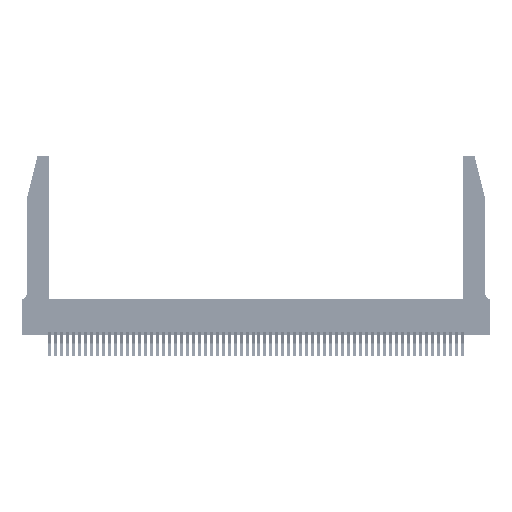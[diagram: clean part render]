
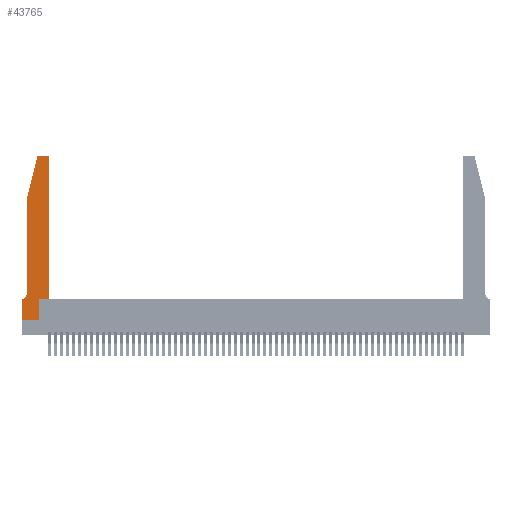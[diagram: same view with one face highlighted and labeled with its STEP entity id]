
A CAD part, top view. The second image highlights one B-rep face of the part: STEP entity #43765.
In plain terms, the highlighted planar face has unit normal (0, 0, 1).
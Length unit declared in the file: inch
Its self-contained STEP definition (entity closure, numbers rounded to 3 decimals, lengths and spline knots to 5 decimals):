
#1650 = CIRCLE ( 'NONE', #48432, 0.07 ) ;
#1701 = CARTESIAN_POINT ( 'NONE',  ( 0.25487, 2.72718, 0.37 ) ) ;
#2907 = VECTOR ( 'NONE', #38109, 39.37008 ) ;
#3611 = LINE ( 'NONE', #40424, #30001 ) ;
#4774 = ORIENTED_EDGE ( 'NONE', *, *, #10449, .T. ) ;
#5428 = VERTEX_POINT ( 'NONE', #1701 ) ;
#5796 = ORIENTED_EDGE ( 'NONE', *, *, #35148, .T. ) ;
#6110 = VECTOR ( 'NONE', #34499, 39.37008 ) ;
#6294 = ORIENTED_EDGE ( 'NONE', *, *, #17720, .T. ) ;
#7890 = VERTEX_POINT ( 'NONE', #23290 ) ;
#7939 = ORIENTED_EDGE ( 'NONE', *, *, #19952, .T. ) ;
#8079 = CARTESIAN_POINT ( 'NONE',  ( 0., 0.35, 0.37 ) ) ;
#8373 = CARTESIAN_POINT ( 'NONE',  ( 0., 0.35, 0.37 ) ) ;
#9248 = VECTOR ( 'NONE', #18853, 39.37008 ) ;
#9257 = AXIS2_PLACEMENT_3D ( 'NONE', #19290, #45790, #23870 ) ;
#10449 = EDGE_CURVE ( 'NONE', #30890, #24434, #25084, .T. ) ;
#11018 = CARTESIAN_POINT ( 'NONE',  ( 0.4505, 0.35, 0.37 ) ) ;
#11156 = VERTEX_POINT ( 'NONE', #47682 ) ;
#12331 = AXIS2_PLACEMENT_3D ( 'NONE', #15056, #23778, #18841 ) ;
#12369 = PLANE ( 'NONE',  #45877 ) ;
#12887 = CARTESIAN_POINT ( 'NONE',  ( 0.4205, 2.75, 0.37 ) ) ;
#13265 = VERTEX_POINT ( 'NONE', #41209 ) ;
#14393 = EDGE_CURVE ( 'NONE', #37479, #23660, #1650, .T. ) ;
#14399 = LINE ( 'NONE', #33569, #2907 ) ;
#14566 = VECTOR ( 'NONE', #15177, 39.37008 ) ;
#14659 = DIRECTION ( 'NONE',  ( 0., -1., 0. ) ) ;
#14742 = ORIENTED_EDGE ( 'NONE', *, *, #29543, .T. ) ;
#15056 = CARTESIAN_POINT ( 'NONE',  ( 0.284, 2.72, 0.37 ) ) ;
#15161 = ORIENTED_EDGE ( 'NONE', *, *, #37620, .T. ) ;
#15177 = DIRECTION ( 'NONE',  ( 0., 1., 0. ) ) ;
#15316 = LINE ( 'NONE', #29468, #33639 ) ;
#15546 = CARTESIAN_POINT ( 'NONE',  ( 0.0755, 2., 0.37 ) ) ;
#15701 = ORIENTED_EDGE ( 'NONE', *, *, #47760, .T. ) ;
#17720 = EDGE_CURVE ( 'NONE', #7890, #37479, #26825, .T. ) ;
#17823 = CARTESIAN_POINT ( 'NONE',  ( 0., 0., 0.37 ) ) ;
#17863 = EDGE_CURVE ( 'NONE', #11156, #40596, #15316, .T. ) ;
#17932 = LINE ( 'NONE', #49998, #14566 ) ;
#18460 = ORIENTED_EDGE ( 'NONE', *, *, #36901, .T. ) ;
#18503 = ORIENTED_EDGE ( 'NONE', *, *, #42354, .T. ) ;
#18841 = DIRECTION ( 'NONE',  ( 1., 0., 0. ) ) ;
#18853 = DIRECTION ( 'NONE',  ( 0., -1., 0. ) ) ;
#19290 = CARTESIAN_POINT ( 'NONE',  ( 0.4205, 2.72, 0.37 ) ) ;
#19952 = EDGE_CURVE ( 'NONE', #23660, #39487, #14399, .T. ) ;
#20032 = EDGE_LOOP ( 'NONE', ( #5796, #18460, #15161, #6294, #37038, #7939, #15701, #4774, #34388, #26425, #14742, #18503 ) ) ;
#20660 = DIRECTION ( 'NONE',  ( 0., 0., 1. ) ) ;
#20765 = CARTESIAN_POINT ( 'NONE',  ( 0.2865, 0.35, 0.37 ) ) ;
#23290 = CARTESIAN_POINT ( 'NONE',  ( 0.0755, 2., 0.37 ) ) ;
#23589 = CARTESIAN_POINT ( 'NONE',  ( 0.0055, 0.35, 0.37 ) ) ;
#23660 = VERTEX_POINT ( 'NONE', #23589 ) ;
#23778 = DIRECTION ( 'NONE',  ( 0., 0., 1. ) ) ;
#23870 = DIRECTION ( 'NONE',  ( 1., 0., 0. ) ) ;
#24434 = VERTEX_POINT ( 'NONE', #51154 ) ;
#25084 = LINE ( 'NONE', #17823, #6110 ) ;
#26360 = VERTEX_POINT ( 'NONE', #12887 ) ;
#26425 = ORIENTED_EDGE ( 'NONE', *, *, #17863, .T. ) ;
#26825 = LINE ( 'NONE', #49326, #9248 ) ;
#28053 = DIRECTION ( 'NONE',  ( -1., 0., 0. ) ) ;
#29468 = CARTESIAN_POINT ( 'NONE',  ( 0.4505, 0.35, 0.37 ) ) ;
#29543 = EDGE_CURVE ( 'NONE', #40596, #13265, #17932, .T. ) ;
#30001 = VECTOR ( 'NONE', #14659, 39.37008 ) ;
#30333 = EDGE_CURVE ( 'NONE', #24434, #11156, #36844, .T. ) ;
#30449 = VECTOR ( 'NONE', #32215, 39.37008 ) ;
#30890 = VERTEX_POINT ( 'NONE', #54794 ) ;
#31772 = VERTEX_POINT ( 'NONE', #43713 ) ;
#32215 = DIRECTION ( 'NONE',  ( -0.239, -0.971, 0. ) ) ;
#33274 = DIRECTION ( 'NONE',  ( 0., 1., 0. ) ) ;
#33569 = CARTESIAN_POINT ( 'NONE',  ( 0.0755, 0.35, 0.37 ) ) ;
#33639 = VECTOR ( 'NONE', #53867, 39.37008 ) ;
#34146 = VECTOR ( 'NONE', #33274, 39.37008 ) ;
#34388 = ORIENTED_EDGE ( 'NONE', *, *, #30333, .T. ) ;
#34499 = DIRECTION ( 'NONE',  ( 1., 0., 0. ) ) ;
#35148 = EDGE_CURVE ( 'NONE', #26360, #31772, #46287, .T. ) ;
#36403 = CARTESIAN_POINT ( 'NONE',  ( 0.0055, 0.42, 0.37 ) ) ;
#36844 = LINE ( 'NONE', #20765, #34146 ) ;
#36901 = EDGE_CURVE ( 'NONE', #31772, #5428, #52225, .T. ) ;
#37038 = ORIENTED_EDGE ( 'NONE', *, *, #14393, .T. ) ;
#37479 = VERTEX_POINT ( 'NONE', #40373 ) ;
#37620 = EDGE_CURVE ( 'NONE', #5428, #7890, #41949, .T. ) ;
#38109 = DIRECTION ( 'NONE',  ( -1., 0., 0. ) ) ;
#39487 = VERTEX_POINT ( 'NONE', #8079 ) ;
#40373 = CARTESIAN_POINT ( 'NONE',  ( 0.0755, 0.42, 0.37 ) ) ;
#40424 = CARTESIAN_POINT ( 'NONE',  ( 0., 0., 0.37 ) ) ;
#40596 = VERTEX_POINT ( 'NONE', #11018 ) ;
#41209 = CARTESIAN_POINT ( 'NONE',  ( 0.4505, 2.72, 0.37 ) ) ;
#41492 = CIRCLE ( 'NONE', #9257, 0.03 ) ;
#41949 = LINE ( 'NONE', #15546, #30449 ) ;
#42354 = EDGE_CURVE ( 'NONE', #13265, #26360, #41492, .T. ) ;
#43713 = CARTESIAN_POINT ( 'NONE',  ( 0.284, 2.75, 0.37 ) ) ;
#43765 = ADVANCED_FACE ( 'NONE', ( #46169 ), #12369, .T. ) ;
#45790 = DIRECTION ( 'NONE',  ( 0., 0., 1. ) ) ;
#45877 = AXIS2_PLACEMENT_3D ( 'NONE', #8373, #20660, #55313 ) ;
#46169 = FACE_OUTER_BOUND ( 'NONE', #20032, .T. ) ;
#46287 = LINE ( 'NONE', #51187, #55820 ) ;
#47682 = CARTESIAN_POINT ( 'NONE',  ( 0.2865, 0.35, 0.37 ) ) ;
#47760 = EDGE_CURVE ( 'NONE', #39487, #30890, #3611, .T. ) ;
#48432 = AXIS2_PLACEMENT_3D ( 'NONE', #36403, #49077, #28053 ) ;
#49077 = DIRECTION ( 'NONE',  ( 0., 0., -1. ) ) ;
#49326 = CARTESIAN_POINT ( 'NONE',  ( 0.0755, 2., 0.37 ) ) ;
#49998 = CARTESIAN_POINT ( 'NONE',  ( 0.4505, 0.35, 0.37 ) ) ;
#51154 = CARTESIAN_POINT ( 'NONE',  ( 0.2865, 0., 0.37 ) ) ;
#51187 = CARTESIAN_POINT ( 'NONE',  ( 0.2605, 2.75, 0.37 ) ) ;
#52225 = CIRCLE ( 'NONE', #12331, 0.03 ) ;
#53867 = DIRECTION ( 'NONE',  ( 1., 0., 0. ) ) ;
#54794 = CARTESIAN_POINT ( 'NONE',  ( 0., 0., 0.37 ) ) ;
#55313 = DIRECTION ( 'NONE',  ( 1., 0., 0. ) ) ;
#55540 = DIRECTION ( 'NONE',  ( -1., 0., 0. ) ) ;
#55820 = VECTOR ( 'NONE', #55540, 39.37008 ) ;
